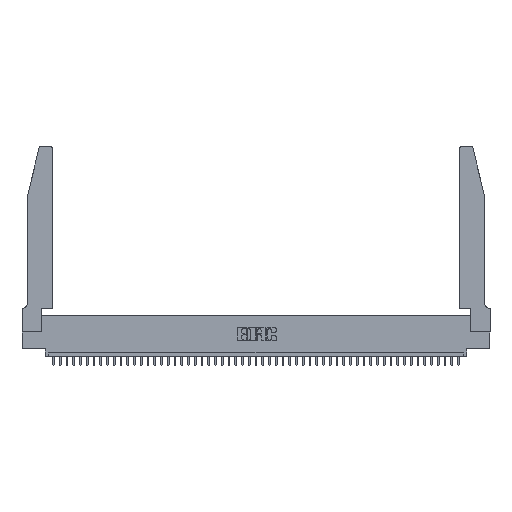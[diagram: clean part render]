
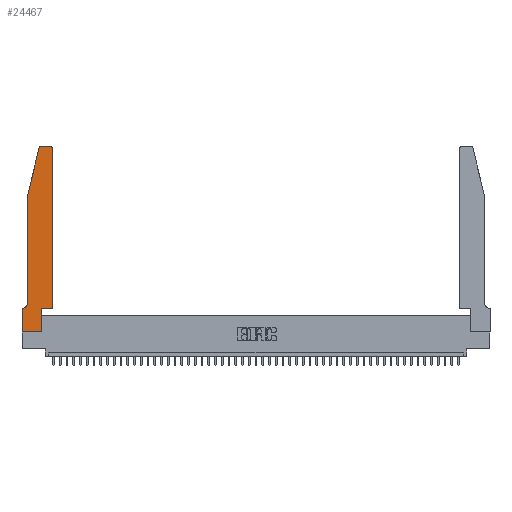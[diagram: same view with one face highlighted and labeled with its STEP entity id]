
A CAD part, top view. The second image highlights one B-rep face of the part: STEP entity #24467.
In plain terms, the highlighted planar face has unit normal (0, 0, 1).
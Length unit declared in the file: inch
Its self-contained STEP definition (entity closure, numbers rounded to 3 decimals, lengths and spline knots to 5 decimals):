
#54 = EDGE_CURVE ( 'NONE', #32928, #30088, #33284, .T. ) ;
#162 = VECTOR ( 'NONE', #36892, 39.37008 ) ;
#844 = CARTESIAN_POINT ( 'NONE',  ( 0.284, 2.75, 0.37 ) ) ;
#1148 = EDGE_CURVE ( 'NONE', #35342, #23860, #15101, .T. ) ;
#1589 = DIRECTION ( 'NONE',  ( -1., 0., 0. ) ) ;
#2551 = EDGE_LOOP ( 'NONE', ( #42036, #45390, #20472, #47572, #5207, #30953, #20381, #40855, #40089, #37703, #15735, #24529 ) ) ;
#3194 = CARTESIAN_POINT ( 'NONE',  ( 0.0755, 2., 0.37 ) ) ;
#4604 = VECTOR ( 'NONE', #19744, 39.37008 ) ;
#5136 = VECTOR ( 'NONE', #39156, 39.37008 ) ;
#5207 = ORIENTED_EDGE ( 'NONE', *, *, #39057, .T. ) ;
#5806 = LINE ( 'NONE', #30507, #4604 ) ;
#6058 = DIRECTION ( 'NONE',  ( 0., 0., -1. ) ) ;
#6525 = VERTEX_POINT ( 'NONE', #12944 ) ;
#6697 = VECTOR ( 'NONE', #23921, 39.37008 ) ;
#7825 = AXIS2_PLACEMENT_3D ( 'NONE', #27361, #31761, #39375 ) ;
#8051 = CIRCLE ( 'NONE', #43579, 0.07 ) ;
#8324 = CARTESIAN_POINT ( 'NONE',  ( 0., 0., 0.37 ) ) ;
#8711 = VERTEX_POINT ( 'NONE', #29363 ) ;
#11542 = CARTESIAN_POINT ( 'NONE',  ( 0.0755, 0.35, 0.37 ) ) ;
#12188 = CARTESIAN_POINT ( 'NONE',  ( 0.4505, 0.35, 0.37 ) ) ;
#12944 = CARTESIAN_POINT ( 'NONE',  ( 0.0755, 0.42, 0.37 ) ) ;
#13287 = VERTEX_POINT ( 'NONE', #23383 ) ;
#13510 = FACE_OUTER_BOUND ( 'NONE', #2551, .T. ) ;
#13820 = VECTOR ( 'NONE', #1589, 39.37008 ) ;
#14710 = DIRECTION ( 'NONE',  ( 0., -1., 0. ) ) ;
#15101 = CIRCLE ( 'NONE', #31382, 0.03 ) ;
#15735 = ORIENTED_EDGE ( 'NONE', *, *, #17007, .T. ) ;
#17007 = EDGE_CURVE ( 'NONE', #13287, #35342, #25331, .T. ) ;
#17500 = EDGE_CURVE ( 'NONE', #26615, #28800, #42114, .T. ) ;
#17640 = CARTESIAN_POINT ( 'NONE',  ( 0.25487, 2.72718, 0.37 ) ) ;
#17777 = CARTESIAN_POINT ( 'NONE',  ( 0.2865, 0., 0.37 ) ) ;
#18389 = LINE ( 'NONE', #11542, #13820 ) ;
#19331 = CARTESIAN_POINT ( 'NONE',  ( 0., 0., 0.37 ) ) ;
#19744 = DIRECTION ( 'NONE',  ( 0., 1., 0. ) ) ;
#19835 = CARTESIAN_POINT ( 'NONE',  ( 0.4505, 0.35, 0.37 ) ) ;
#20381 = ORIENTED_EDGE ( 'NONE', *, *, #17500, .T. ) ;
#20470 = VECTOR ( 'NONE', #44642, 39.37008 ) ;
#20472 = ORIENTED_EDGE ( 'NONE', *, *, #54, .T. ) ;
#20508 = EDGE_CURVE ( 'NONE', #45231, #32928, #23840, .T. ) ;
#21020 = DIRECTION ( 'NONE',  ( -1., 0., 0. ) ) ;
#21574 = VECTOR ( 'NONE', #14710, 39.37008 ) ;
#23383 = CARTESIAN_POINT ( 'NONE',  ( 0.4505, 0.35, 0.37 ) ) ;
#23840 = CIRCLE ( 'NONE', #7825, 0.03 ) ;
#23860 = VERTEX_POINT ( 'NONE', #43190 ) ;
#23921 = DIRECTION ( 'NONE',  ( 0., 1., 0. ) ) ;
#24467 = ADVANCED_FACE ( 'NONE', ( #13510 ), #31259, .T. ) ;
#24529 = ORIENTED_EDGE ( 'NONE', *, *, #1148, .T. ) ;
#24705 = VECTOR ( 'NONE', #35835, 39.37008 ) ;
#24860 = EDGE_CURVE ( 'NONE', #8711, #13287, #46061, .T. ) ;
#25331 = LINE ( 'NONE', #19835, #6697 ) ;
#25968 = EDGE_CURVE ( 'NONE', #28800, #46270, #39504, .T. ) ;
#26276 = VECTOR ( 'NONE', #43127, 39.37008 ) ;
#26615 = VERTEX_POINT ( 'NONE', #33678 ) ;
#27241 = EDGE_CURVE ( 'NONE', #27654, #26615, #18389, .T. ) ;
#27361 = CARTESIAN_POINT ( 'NONE',  ( 0.284, 2.72, 0.37 ) ) ;
#27364 = DIRECTION ( 'NONE',  ( 1., 0., 0. ) ) ;
#27654 = VERTEX_POINT ( 'NONE', #44962 ) ;
#28573 = EDGE_CURVE ( 'NONE', #23860, #45231, #39824, .T. ) ;
#28800 = VERTEX_POINT ( 'NONE', #8324 ) ;
#29186 = CARTESIAN_POINT ( 'NONE',  ( 0.0755, 2., 0.37 ) ) ;
#29363 = CARTESIAN_POINT ( 'NONE',  ( 0.2865, 0.35, 0.37 ) ) ;
#30088 = VERTEX_POINT ( 'NONE', #35077 ) ;
#30507 = CARTESIAN_POINT ( 'NONE',  ( 0.2865, 0.35, 0.37 ) ) ;
#30953 = ORIENTED_EDGE ( 'NONE', *, *, #27241, .T. ) ;
#31259 = PLANE ( 'NONE',  #33787 ) ;
#31382 = AXIS2_PLACEMENT_3D ( 'NONE', #45475, #34782, #38142 ) ;
#31761 = DIRECTION ( 'NONE',  ( 0., 0., 1. ) ) ;
#32928 = VERTEX_POINT ( 'NONE', #17640 ) ;
#33284 = LINE ( 'NONE', #3194, #20470 ) ;
#33444 = CARTESIAN_POINT ( 'NONE',  ( 0.2605, 2.75, 0.37 ) ) ;
#33678 = CARTESIAN_POINT ( 'NONE',  ( 0., 0.35, 0.37 ) ) ;
#33787 = AXIS2_PLACEMENT_3D ( 'NONE', #42306, #34860, #27364 ) ;
#33797 = LINE ( 'NONE', #29186, #21574 ) ;
#34782 = DIRECTION ( 'NONE',  ( 0., 0., 1. ) ) ;
#34860 = DIRECTION ( 'NONE',  ( 0., 0., 1. ) ) ;
#35077 = CARTESIAN_POINT ( 'NONE',  ( 0.0755, 2., 0.37 ) ) ;
#35342 = VERTEX_POINT ( 'NONE', #42593 ) ;
#35835 = DIRECTION ( 'NONE',  ( 0., -1., 0. ) ) ;
#36892 = DIRECTION ( 'NONE',  ( -1., 0., 0. ) ) ;
#37440 = EDGE_CURVE ( 'NONE', #30088, #6525, #33797, .T. ) ;
#37703 = ORIENTED_EDGE ( 'NONE', *, *, #24860, .T. ) ;
#38142 = DIRECTION ( 'NONE',  ( 1., 0., 0. ) ) ;
#39057 = EDGE_CURVE ( 'NONE', #6525, #27654, #8051, .T. ) ;
#39156 = DIRECTION ( 'NONE',  ( 1., 0., 0. ) ) ;
#39375 = DIRECTION ( 'NONE',  ( 1., 0., 0. ) ) ;
#39504 = LINE ( 'NONE', #46162, #5136 ) ;
#39824 = LINE ( 'NONE', #33444, #162 ) ;
#40089 = ORIENTED_EDGE ( 'NONE', *, *, #41672, .T. ) ;
#40855 = ORIENTED_EDGE ( 'NONE', *, *, #25968, .T. ) ;
#41672 = EDGE_CURVE ( 'NONE', #46270, #8711, #5806, .T. ) ;
#42036 = ORIENTED_EDGE ( 'NONE', *, *, #28573, .T. ) ;
#42114 = LINE ( 'NONE', #19331, #24705 ) ;
#42306 = CARTESIAN_POINT ( 'NONE',  ( 0., 0.35, 0.37 ) ) ;
#42593 = CARTESIAN_POINT ( 'NONE',  ( 0.4505, 2.72, 0.37 ) ) ;
#43127 = DIRECTION ( 'NONE',  ( 1., 0., 0. ) ) ;
#43168 = CARTESIAN_POINT ( 'NONE',  ( 0.0055, 0.42, 0.37 ) ) ;
#43190 = CARTESIAN_POINT ( 'NONE',  ( 0.4205, 2.75, 0.37 ) ) ;
#43579 = AXIS2_PLACEMENT_3D ( 'NONE', #43168, #6058, #21020 ) ;
#44642 = DIRECTION ( 'NONE',  ( -0.239, -0.971, 0. ) ) ;
#44962 = CARTESIAN_POINT ( 'NONE',  ( 0.0055, 0.35, 0.37 ) ) ;
#45231 = VERTEX_POINT ( 'NONE', #844 ) ;
#45390 = ORIENTED_EDGE ( 'NONE', *, *, #20508, .T. ) ;
#45475 = CARTESIAN_POINT ( 'NONE',  ( 0.4205, 2.72, 0.37 ) ) ;
#46061 = LINE ( 'NONE', #12188, #26276 ) ;
#46162 = CARTESIAN_POINT ( 'NONE',  ( 0., 0., 0.37 ) ) ;
#46270 = VERTEX_POINT ( 'NONE', #17777 ) ;
#47572 = ORIENTED_EDGE ( 'NONE', *, *, #37440, .T. ) ;
